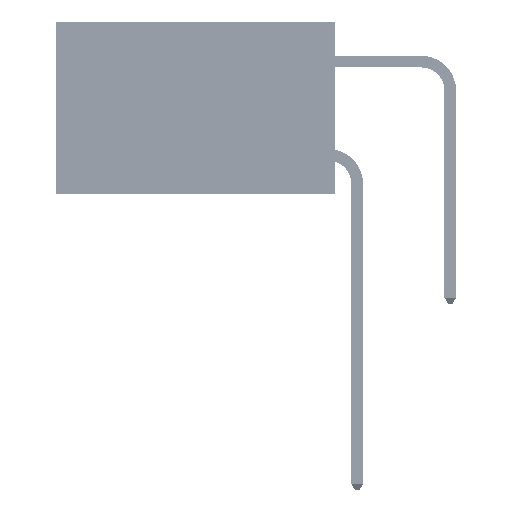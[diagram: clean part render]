
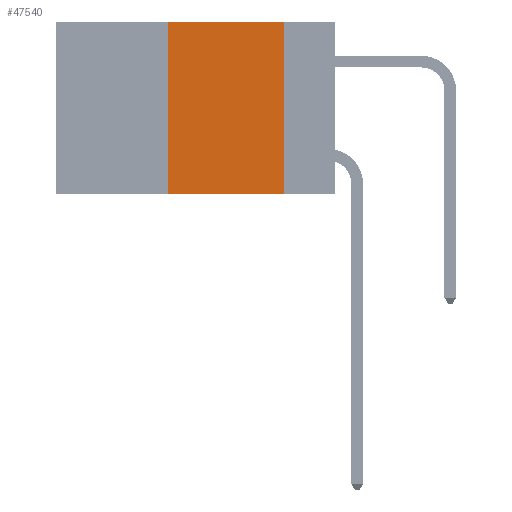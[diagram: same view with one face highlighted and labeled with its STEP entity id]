
A CAD part, left-side view. The second image highlights one B-rep face of the part: STEP entity #47540.
In plain terms, the highlighted planar face has unit normal (-1, 0, 0).
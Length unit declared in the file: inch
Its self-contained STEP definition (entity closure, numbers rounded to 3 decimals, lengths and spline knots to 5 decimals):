
#56 = LINE ( 'NONE', #40050, #16279 ) ;
#66 = CARTESIAN_POINT ( 'NONE',  ( 0., 0.11, -0.37 ) ) ;
#705 = CARTESIAN_POINT ( 'NONE',  ( 0., 0.6, 0. ) ) ;
#1108 = VERTEX_POINT ( 'NONE', #14660 ) ;
#2578 = EDGE_CURVE ( 'NONE', #12523, #29835, #34826, .T. ) ;
#4178 = VECTOR ( 'NONE', #40917, 39.37008 ) ;
#4789 = VECTOR ( 'NONE', #14100, 39.37008 ) ;
#9681 = ORIENTED_EDGE ( 'NONE', *, *, #18778, .T. ) ;
#12090 = PLANE ( 'NONE',  #31575 ) ;
#12523 = VERTEX_POINT ( 'NONE', #46489 ) ;
#12876 = ORIENTED_EDGE ( 'NONE', *, *, #20775, .F. ) ;
#14100 = DIRECTION ( 'NONE',  ( 0., -1., 0. ) ) ;
#14660 = CARTESIAN_POINT ( 'NONE',  ( 0., 0.36, 0. ) ) ;
#16279 = VECTOR ( 'NONE', #25236, 39.37008 ) ;
#17507 = DIRECTION ( 'NONE',  ( 0., 0., 1. ) ) ;
#18488 = FACE_OUTER_BOUND ( 'NONE', #43084, .T. ) ;
#18778 = EDGE_CURVE ( 'NONE', #46388, #29835, #56, .T. ) ;
#20775 = EDGE_CURVE ( 'NONE', #46388, #1108, #39487, .T. ) ;
#23792 = EDGE_CURVE ( 'NONE', #1108, #12523, #31785, .T. ) ;
#25236 = DIRECTION ( 'NONE',  ( 0., -1., 0. ) ) ;
#25397 = CARTESIAN_POINT ( 'NONE',  ( 0., 0.11, 0. ) ) ;
#26906 = ORIENTED_EDGE ( 'NONE', *, *, #2578, .F. ) ;
#27547 = DIRECTION ( 'NONE',  ( 1., 0., 0. ) ) ;
#29835 = VERTEX_POINT ( 'NONE', #66 ) ;
#31376 = DIRECTION ( 'NONE',  ( 0., 0., -1. ) ) ;
#31575 = AXIS2_PLACEMENT_3D ( 'NONE', #705, #27547, #31376 ) ;
#31785 = LINE ( 'NONE', #47880, #4789 ) ;
#34826 = LINE ( 'NONE', #25397, #4178 ) ;
#39487 = LINE ( 'NONE', #40533, #41274 ) ;
#40050 = CARTESIAN_POINT ( 'NONE',  ( 0., 0.6, -0.37 ) ) ;
#40073 = ORIENTED_EDGE ( 'NONE', *, *, #23792, .F. ) ;
#40533 = CARTESIAN_POINT ( 'NONE',  ( 0., 0.36, 0. ) ) ;
#40917 = DIRECTION ( 'NONE',  ( 0., 0., -1. ) ) ;
#41274 = VECTOR ( 'NONE', #17507, 39.37008 ) ;
#43084 = EDGE_LOOP ( 'NONE', ( #26906, #40073, #12876, #9681 ) ) ;
#43564 = CARTESIAN_POINT ( 'NONE',  ( 0., 0.36, -0.37 ) ) ;
#46388 = VERTEX_POINT ( 'NONE', #43564 ) ;
#46489 = CARTESIAN_POINT ( 'NONE',  ( 0., 0.11, 0. ) ) ;
#47540 = ADVANCED_FACE ( 'NONE', ( #18488 ), #12090, .F. ) ;
#47880 = CARTESIAN_POINT ( 'NONE',  ( 0., 0.6, 0. ) ) ;
